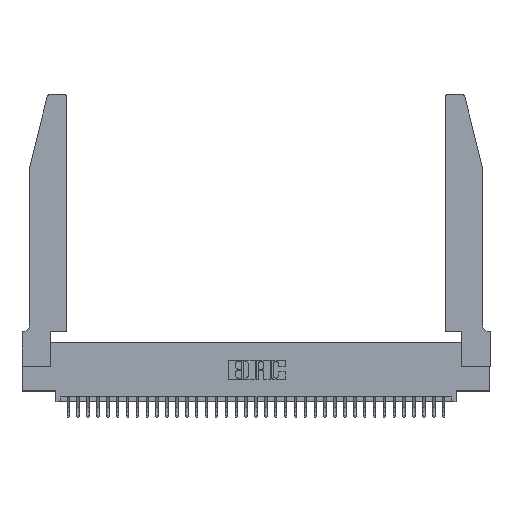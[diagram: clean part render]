
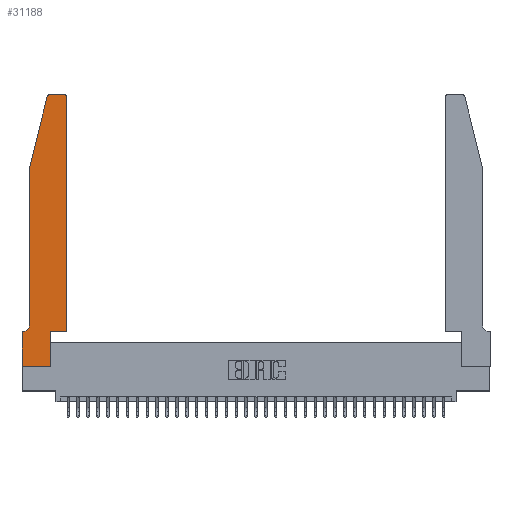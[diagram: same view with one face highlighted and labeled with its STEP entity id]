
A CAD part, top view. The second image highlights one B-rep face of the part: STEP entity #31188.
In plain terms, the highlighted planar face has unit normal (0, 0, 1).
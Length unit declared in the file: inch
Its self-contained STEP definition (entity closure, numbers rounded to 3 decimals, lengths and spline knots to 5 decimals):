
#65 = DIRECTION ( 'NONE',  ( 0., -1., 0. ) ) ;
#1359 = ORIENTED_EDGE ( 'NONE', *, *, #32696, .T. ) ;
#2386 = CARTESIAN_POINT ( 'NONE',  ( 0., 0.35, 0.37 ) ) ;
#2973 = VECTOR ( 'NONE', #65, 39.37008 ) ;
#3200 = LINE ( 'NONE', #31507, #26309 ) ;
#3203 = ORIENTED_EDGE ( 'NONE', *, *, #35718, .T. ) ;
#3219 = DIRECTION ( 'NONE',  ( 0., 0., 1. ) ) ;
#4061 = EDGE_CURVE ( 'NONE', #28679, #7071, #22799, .T. ) ;
#4936 = CARTESIAN_POINT ( 'NONE',  ( 0.0055, 0.35, 0.37 ) ) ;
#5068 = CARTESIAN_POINT ( 'NONE',  ( 0.4505, 0.35, 0.37 ) ) ;
#5101 = AXIS2_PLACEMENT_3D ( 'NONE', #20005, #3219, #22760 ) ;
#5605 = LINE ( 'NONE', #31044, #19571 ) ;
#5917 = CARTESIAN_POINT ( 'NONE',  ( 0.284, 2.75, 0.37 ) ) ;
#6504 = DIRECTION ( 'NONE',  ( 1., 0., 0. ) ) ;
#6702 = CARTESIAN_POINT ( 'NONE',  ( 0.4205, 2.75, 0.37 ) ) ;
#6920 = CARTESIAN_POINT ( 'NONE',  ( 0.2605, 2.75, 0.37 ) ) ;
#7071 = VERTEX_POINT ( 'NONE', #33886 ) ;
#7207 = EDGE_CURVE ( 'NONE', #28699, #24633, #8281, .T. ) ;
#7285 = CARTESIAN_POINT ( 'NONE',  ( 0.0755, 2., 0.37 ) ) ;
#7965 = VERTEX_POINT ( 'NONE', #26853 ) ;
#8086 = DIRECTION ( 'NONE',  ( 1., 0., 0. ) ) ;
#8120 = EDGE_CURVE ( 'NONE', #33206, #29055, #11400, .T. ) ;
#8212 = CARTESIAN_POINT ( 'NONE',  ( 0.4205, 2.72, 0.37 ) ) ;
#8281 = LINE ( 'NONE', #6920, #22133 ) ;
#8595 = ORIENTED_EDGE ( 'NONE', *, *, #26290, .T. ) ;
#8656 = DIRECTION ( 'NONE',  ( 0., 1., 0. ) ) ;
#9365 = FACE_OUTER_BOUND ( 'NONE', #23708, .T. ) ;
#9791 = CARTESIAN_POINT ( 'NONE',  ( 0.4505, 2.72, 0.37 ) ) ;
#10714 = CARTESIAN_POINT ( 'NONE',  ( 0.25487, 2.72718, 0.37 ) ) ;
#11079 = DIRECTION ( 'NONE',  ( 1., 0., 0. ) ) ;
#11400 = LINE ( 'NONE', #27452, #30738 ) ;
#11687 = ORIENTED_EDGE ( 'NONE', *, *, #19617, .T. ) ;
#11910 = VECTOR ( 'NONE', #8656, 39.37008 ) ;
#12398 = VERTEX_POINT ( 'NONE', #2386 ) ;
#12845 = LINE ( 'NONE', #5068, #33921 ) ;
#13382 = ORIENTED_EDGE ( 'NONE', *, *, #7207, .T. ) ;
#13526 = VERTEX_POINT ( 'NONE', #10714 ) ;
#15161 = EDGE_CURVE ( 'NONE', #13526, #28679, #3200, .T. ) ;
#15490 = CARTESIAN_POINT ( 'NONE',  ( 0.0055, 0.42, 0.37 ) ) ;
#16868 = EDGE_CURVE ( 'NONE', #24633, #13526, #24004, .T. ) ;
#17271 = ORIENTED_EDGE ( 'NONE', *, *, #8120, .T. ) ;
#17581 = PLANE ( 'NONE',  #33554 ) ;
#17712 = ORIENTED_EDGE ( 'NONE', *, *, #29761, .T. ) ;
#17775 = CARTESIAN_POINT ( 'NONE',  ( 0.0755, 2., 0.37 ) ) ;
#18029 = LINE ( 'NONE', #18795, #19772 ) ;
#18263 = DIRECTION ( 'NONE',  ( -1., 0., 0. ) ) ;
#18795 = CARTESIAN_POINT ( 'NONE',  ( 0.0755, 0.35, 0.37 ) ) ;
#19001 = CIRCLE ( 'NONE', #31466, 0.07 ) ;
#19038 = VERTEX_POINT ( 'NONE', #20158 ) ;
#19571 = VECTOR ( 'NONE', #28283, 39.37008 ) ;
#19617 = EDGE_CURVE ( 'NONE', #7965, #19038, #5605, .T. ) ;
#19772 = VECTOR ( 'NONE', #35256, 39.37008 ) ;
#20005 = CARTESIAN_POINT ( 'NONE',  ( 0.284, 2.72, 0.37 ) ) ;
#20158 = CARTESIAN_POINT ( 'NONE',  ( 0.4505, 0.35, 0.37 ) ) ;
#20575 = DIRECTION ( 'NONE',  ( -0.239, -0.971, 0. ) ) ;
#21143 = ORIENTED_EDGE ( 'NONE', *, *, #25636, .T. ) ;
#22133 = VECTOR ( 'NONE', #28809, 39.37008 ) ;
#22587 = CARTESIAN_POINT ( 'NONE',  ( 0., 0., 0.37 ) ) ;
#22760 = DIRECTION ( 'NONE',  ( 1., 0., 0. ) ) ;
#22799 = LINE ( 'NONE', #7285, #29254 ) ;
#23111 = DIRECTION ( 'NONE',  ( 0., 0., 1. ) ) ;
#23708 = EDGE_LOOP ( 'NONE', ( #13382, #29721, #31438, #25012, #25871, #21143, #1359, #17271, #3203, #11687, #8595, #17712 ) ) ;
#23893 = DIRECTION ( 'NONE',  ( 0., -1., 0. ) ) ;
#24004 = CIRCLE ( 'NONE', #5101, 0.03 ) ;
#24247 = EDGE_CURVE ( 'NONE', #7071, #24412, #19001, .T. ) ;
#24376 = LINE ( 'NONE', #22587, #2973 ) ;
#24412 = VERTEX_POINT ( 'NONE', #4936 ) ;
#24633 = VERTEX_POINT ( 'NONE', #5917 ) ;
#25012 = ORIENTED_EDGE ( 'NONE', *, *, #4061, .T. ) ;
#25103 = CARTESIAN_POINT ( 'NONE',  ( 0.2865, 0., 0.37 ) ) ;
#25233 = CARTESIAN_POINT ( 'NONE',  ( 0.2865, 0.35, 0.37 ) ) ;
#25636 = EDGE_CURVE ( 'NONE', #24412, #12398, #18029, .T. ) ;
#25871 = ORIENTED_EDGE ( 'NONE', *, *, #24247, .T. ) ;
#26290 = EDGE_CURVE ( 'NONE', #19038, #28771, #12845, .T. ) ;
#26309 = VECTOR ( 'NONE', #20575, 39.37008 ) ;
#26853 = CARTESIAN_POINT ( 'NONE',  ( 0.2865, 0.35, 0.37 ) ) ;
#27452 = CARTESIAN_POINT ( 'NONE',  ( 0., 0., 0.37 ) ) ;
#27554 = DIRECTION ( 'NONE',  ( 0., 0., 1. ) ) ;
#28283 = DIRECTION ( 'NONE',  ( 1., 0., 0. ) ) ;
#28527 = CARTESIAN_POINT ( 'NONE',  ( 0., 0.35, 0.37 ) ) ;
#28679 = VERTEX_POINT ( 'NONE', #17775 ) ;
#28699 = VERTEX_POINT ( 'NONE', #6702 ) ;
#28771 = VERTEX_POINT ( 'NONE', #9791 ) ;
#28809 = DIRECTION ( 'NONE',  ( -1., 0., 0. ) ) ;
#28902 = AXIS2_PLACEMENT_3D ( 'NONE', #8212, #27554, #11079 ) ;
#29055 = VERTEX_POINT ( 'NONE', #25103 ) ;
#29254 = VECTOR ( 'NONE', #23893, 39.37008 ) ;
#29721 = ORIENTED_EDGE ( 'NONE', *, *, #16868, .T. ) ;
#29761 = EDGE_CURVE ( 'NONE', #28771, #28699, #30595, .T. ) ;
#30595 = CIRCLE ( 'NONE', #28902, 0.03 ) ;
#30738 = VECTOR ( 'NONE', #8086, 39.37008 ) ;
#31044 = CARTESIAN_POINT ( 'NONE',  ( 0.4505, 0.35, 0.37 ) ) ;
#31188 = ADVANCED_FACE ( 'NONE', ( #9365 ), #17581, .T. ) ;
#31438 = ORIENTED_EDGE ( 'NONE', *, *, #15161, .T. ) ;
#31466 = AXIS2_PLACEMENT_3D ( 'NONE', #15490, #34745, #18263 ) ;
#31507 = CARTESIAN_POINT ( 'NONE',  ( 0.0755, 2., 0.37 ) ) ;
#32696 = EDGE_CURVE ( 'NONE', #12398, #33206, #24376, .T. ) ;
#32794 = DIRECTION ( 'NONE',  ( 0., 1., 0. ) ) ;
#32988 = LINE ( 'NONE', #25233, #11910 ) ;
#33009 = CARTESIAN_POINT ( 'NONE',  ( 0., 0., 0.37 ) ) ;
#33206 = VERTEX_POINT ( 'NONE', #33009 ) ;
#33554 = AXIS2_PLACEMENT_3D ( 'NONE', #28527, #23111, #6504 ) ;
#33886 = CARTESIAN_POINT ( 'NONE',  ( 0.0755, 0.42, 0.37 ) ) ;
#33921 = VECTOR ( 'NONE', #32794, 39.37008 ) ;
#34745 = DIRECTION ( 'NONE',  ( 0., 0., -1. ) ) ;
#35256 = DIRECTION ( 'NONE',  ( -1., 0., 0. ) ) ;
#35718 = EDGE_CURVE ( 'NONE', #29055, #7965, #32988, .T. ) ;
